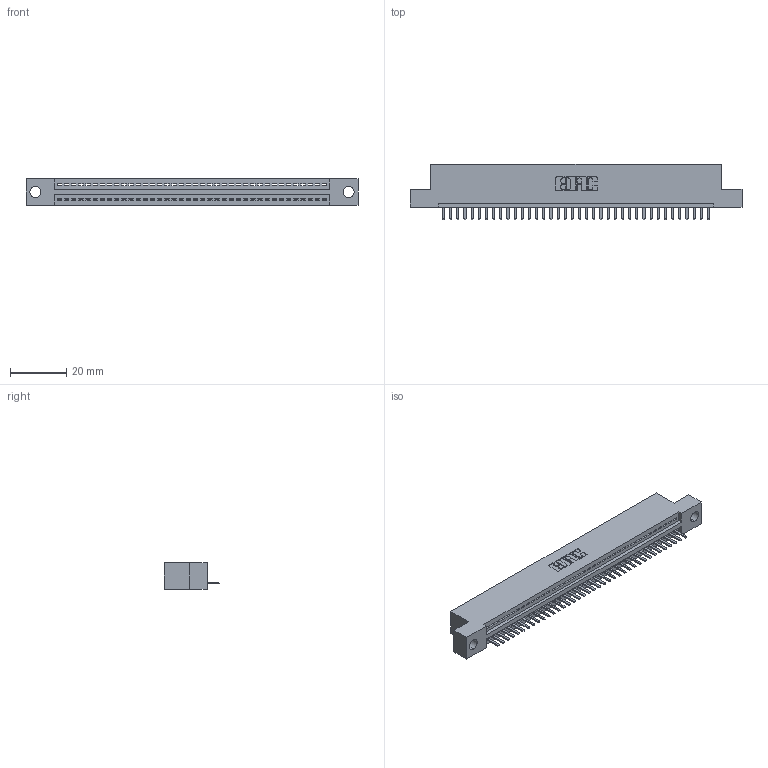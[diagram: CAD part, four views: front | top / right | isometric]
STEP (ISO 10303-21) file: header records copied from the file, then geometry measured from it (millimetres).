
FILE_DESCRIPTION (( 'STEP AP203' ), '1' );
FILE_NAME ('345-038-520-104.STEP', '2019-10-08T02:49:14', ( '' ), ( '' ), 'SwSTEP 2.0', 'SolidWorks 2016', '' );
FILE_SCHEMA (( 'CONFIG_CONTROL_DESIGN' ));
Length unit declared in the file: inch
Products named in the file (3): 345 Part_Flush Mounting Lugs - 0.156 Dia-TH; 345-292-001_345-293-120; 345-038-520-104
Assembly tree (39 placements, depth 2):
  345-038-520-104
    345 Part_Flush Mounting Lugs - 0.156 Dia-TH
    345-292-001_345-293-120  x38
Bounding box: 117.73 x 19.68 x 9.4 mm (x, y, z)
Volume: 10952.1 mm3; surface area: 13951.1 mm2
Topology: 39 solids, 39 shells, 2482 faces, 7333 edges, 4786 vertices
Faces by surface type: plane 1676, cylinder 806
Entity records: 29255 total; most frequent: CARTESIAN_POINT 5086, ORIENTED_EDGE 5046, DIRECTION 4435, EDGE_CURVE 2523, LINE 2235, VECTOR 2235, VERTEX_POINT 1678, AXIS2_PLACEMENT_3D 1100
